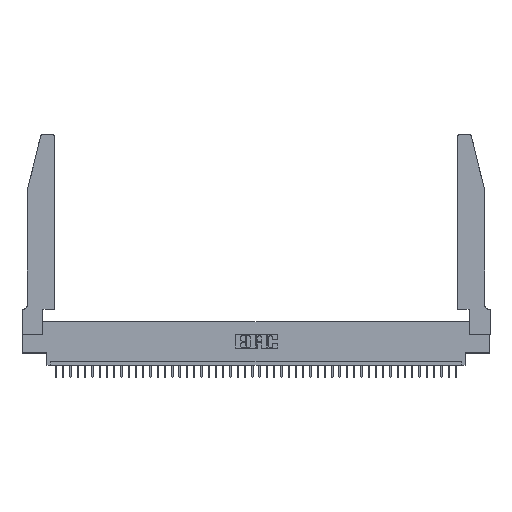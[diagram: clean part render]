
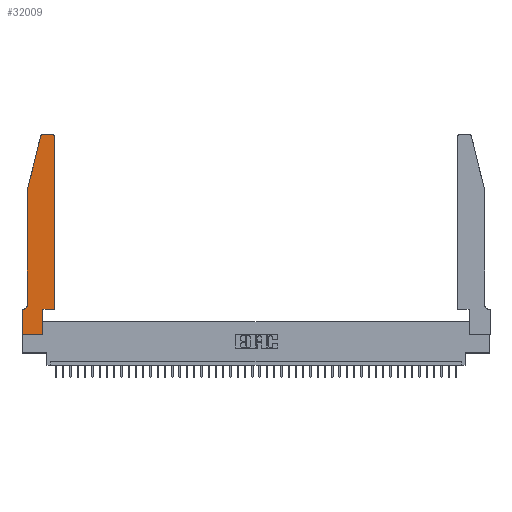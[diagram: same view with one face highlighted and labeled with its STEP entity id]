
A CAD part, top view. The second image highlights one B-rep face of the part: STEP entity #32009.
In plain terms, the highlighted planar face has unit normal (0, 0, 1).
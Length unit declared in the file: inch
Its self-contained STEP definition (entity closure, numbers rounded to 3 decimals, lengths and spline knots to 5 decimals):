
#18 = CARTESIAN_POINT ( 'NONE',  ( 0.0755, 0.42, 0.37 ) ) ;
#1356 = CIRCLE ( 'NONE', #8818, 0.07 ) ;
#1361 = EDGE_CURVE ( 'NONE', #44938, #2321, #7602, .T. ) ;
#1461 = CARTESIAN_POINT ( 'NONE',  ( 0., 0.35, 0.37 ) ) ;
#2094 = CARTESIAN_POINT ( 'NONE',  ( 0.0755, 0.35, 0.37 ) ) ;
#2321 = VERTEX_POINT ( 'NONE', #21608 ) ;
#2689 = VERTEX_POINT ( 'NONE', #36999 ) ;
#2797 = ORIENTED_EDGE ( 'NONE', *, *, #9534, .T. ) ;
#4117 = AXIS2_PLACEMENT_3D ( 'NONE', #1461, #36749, #15804 ) ;
#5917 = CARTESIAN_POINT ( 'NONE',  ( 0.4505, 2.72, 0.37 ) ) ;
#7086 = EDGE_CURVE ( 'NONE', #2689, #9109, #42545, .T. ) ;
#7531 = DIRECTION ( 'NONE',  ( 1., 0., 0. ) ) ;
#7602 = LINE ( 'NONE', #31807, #38711 ) ;
#7651 = EDGE_CURVE ( 'NONE', #26557, #43813, #8145, .T. ) ;
#8145 = LINE ( 'NONE', #15179, #40892 ) ;
#8818 = AXIS2_PLACEMENT_3D ( 'NONE', #43411, #18989, #39770 ) ;
#8921 = ORIENTED_EDGE ( 'NONE', *, *, #43146, .T. ) ;
#9109 = VERTEX_POINT ( 'NONE', #40360 ) ;
#9534 = EDGE_CURVE ( 'NONE', #9109, #19603, #30904, .T. ) ;
#10351 = CARTESIAN_POINT ( 'NONE',  ( 0.284, 2.75, 0.37 ) ) ;
#10446 = CARTESIAN_POINT ( 'NONE',  ( 0.4205, 2.75, 0.37 ) ) ;
#10692 = DIRECTION ( 'NONE',  ( 1., 0., 0. ) ) ;
#11407 = VECTOR ( 'NONE', #44811, 39.37008 ) ;
#11962 = ORIENTED_EDGE ( 'NONE', *, *, #36521, .T. ) ;
#12102 = EDGE_LOOP ( 'NONE', ( #14513, #35256, #32647, #8921, #28893, #36883, #13601, #25697, #11962, #14134, #2797, #15555 ) ) ;
#12489 = EDGE_CURVE ( 'NONE', #29312, #44938, #43324, .T. ) ;
#13601 = ORIENTED_EDGE ( 'NONE', *, *, #19888, .T. ) ;
#14099 = DIRECTION ( 'NONE',  ( 0., -1., 0. ) ) ;
#14134 = ORIENTED_EDGE ( 'NONE', *, *, #7086, .T. ) ;
#14513 = ORIENTED_EDGE ( 'NONE', *, *, #42113, .T. ) ;
#15005 = CARTESIAN_POINT ( 'NONE',  ( 0., 0., 0.37 ) ) ;
#15179 = CARTESIAN_POINT ( 'NONE',  ( 0., 0., 0.37 ) ) ;
#15311 = VERTEX_POINT ( 'NONE', #18 ) ;
#15555 = ORIENTED_EDGE ( 'NONE', *, *, #31331, .T. ) ;
#15804 = DIRECTION ( 'NONE',  ( 1., 0., 0. ) ) ;
#15891 = VERTEX_POINT ( 'NONE', #38110 ) ;
#15934 = DIRECTION ( 'NONE',  ( 0., 0., 1. ) ) ;
#16009 = CARTESIAN_POINT ( 'NONE',  ( 0.4505, 0.35, 0.37 ) ) ;
#16057 = LINE ( 'NONE', #15005, #42832 ) ;
#17105 = VECTOR ( 'NONE', #23163, 39.37008 ) ;
#17868 = DIRECTION ( 'NONE',  ( 0., 0., 1. ) ) ;
#18566 = DIRECTION ( 'NONE',  ( 1., 0., 0. ) ) ;
#18989 = DIRECTION ( 'NONE',  ( 0., 0., -1. ) ) ;
#19302 = VECTOR ( 'NONE', #24880, 39.37008 ) ;
#19389 = CARTESIAN_POINT ( 'NONE',  ( 0.0055, 0.35, 0.37 ) ) ;
#19603 = VERTEX_POINT ( 'NONE', #5917 ) ;
#19888 = EDGE_CURVE ( 'NONE', #15891, #26557, #16057, .T. ) ;
#20320 = EDGE_CURVE ( 'NONE', #27628, #15891, #25340, .T. ) ;
#21608 = CARTESIAN_POINT ( 'NONE',  ( 0.0755, 2., 0.37 ) ) ;
#22881 = LINE ( 'NONE', #26991, #11407 ) ;
#23163 = DIRECTION ( 'NONE',  ( -1., 0., 0. ) ) ;
#23839 = CARTESIAN_POINT ( 'NONE',  ( 0.2605, 2.75, 0.37 ) ) ;
#24000 = VERTEX_POINT ( 'NONE', #10446 ) ;
#24753 = CARTESIAN_POINT ( 'NONE',  ( 0.4505, 0.35, 0.37 ) ) ;
#24880 = DIRECTION ( 'NONE',  ( 0., 1., 0. ) ) ;
#25015 = CARTESIAN_POINT ( 'NONE',  ( 0.2865, 0.35, 0.37 ) ) ;
#25340 = LINE ( 'NONE', #2094, #17105 ) ;
#25630 = VECTOR ( 'NONE', #10692, 39.37008 ) ;
#25697 = ORIENTED_EDGE ( 'NONE', *, *, #7651, .T. ) ;
#25991 = VECTOR ( 'NONE', #40623, 39.37008 ) ;
#26242 = PLANE ( 'NONE',  #4117 ) ;
#26528 = DIRECTION ( 'NONE',  ( 1., 0., 0. ) ) ;
#26557 = VERTEX_POINT ( 'NONE', #40274 ) ;
#26742 = CARTESIAN_POINT ( 'NONE',  ( 0.2865, 0., 0.37 ) ) ;
#26991 = CARTESIAN_POINT ( 'NONE',  ( 0.0755, 2., 0.37 ) ) ;
#27628 = VERTEX_POINT ( 'NONE', #19389 ) ;
#28893 = ORIENTED_EDGE ( 'NONE', *, *, #44925, .T. ) ;
#29198 = AXIS2_PLACEMENT_3D ( 'NONE', #39396, #17868, #7531 ) ;
#29312 = VERTEX_POINT ( 'NONE', #10351 ) ;
#29405 = CARTESIAN_POINT ( 'NONE',  ( 0.25487, 2.72718, 0.37 ) ) ;
#30904 = LINE ( 'NONE', #16009, #25991 ) ;
#31331 = EDGE_CURVE ( 'NONE', #19603, #24000, #36213, .T. ) ;
#31357 = DIRECTION ( 'NONE',  ( -1., 0., 0. ) ) ;
#31807 = CARTESIAN_POINT ( 'NONE',  ( 0.0755, 2., 0.37 ) ) ;
#32009 = ADVANCED_FACE ( 'NONE', ( #37848 ), #26242, .T. ) ;
#32647 = ORIENTED_EDGE ( 'NONE', *, *, #1361, .T. ) ;
#33020 = VECTOR ( 'NONE', #31357, 39.37008 ) ;
#33562 = LINE ( 'NONE', #23839, #33020 ) ;
#35256 = ORIENTED_EDGE ( 'NONE', *, *, #12489, .T. ) ;
#36213 = CIRCLE ( 'NONE', #36898, 0.03 ) ;
#36521 = EDGE_CURVE ( 'NONE', #43813, #2689, #42244, .T. ) ;
#36749 = DIRECTION ( 'NONE',  ( 0., 0., 1. ) ) ;
#36883 = ORIENTED_EDGE ( 'NONE', *, *, #20320, .T. ) ;
#36898 = AXIS2_PLACEMENT_3D ( 'NONE', #43903, #15934, #26528 ) ;
#36999 = CARTESIAN_POINT ( 'NONE',  ( 0.2865, 0.35, 0.37 ) ) ;
#37848 = FACE_OUTER_BOUND ( 'NONE', #12102, .T. ) ;
#38110 = CARTESIAN_POINT ( 'NONE',  ( 0., 0.35, 0.37 ) ) ;
#38711 = VECTOR ( 'NONE', #43343, 39.37008 ) ;
#39396 = CARTESIAN_POINT ( 'NONE',  ( 0.284, 2.72, 0.37 ) ) ;
#39770 = DIRECTION ( 'NONE',  ( -1., 0., 0. ) ) ;
#40274 = CARTESIAN_POINT ( 'NONE',  ( 0., 0., 0.37 ) ) ;
#40360 = CARTESIAN_POINT ( 'NONE',  ( 0.4505, 0.35, 0.37 ) ) ;
#40623 = DIRECTION ( 'NONE',  ( 0., 1., 0. ) ) ;
#40892 = VECTOR ( 'NONE', #18566, 39.37008 ) ;
#42113 = EDGE_CURVE ( 'NONE', #24000, #29312, #33562, .T. ) ;
#42244 = LINE ( 'NONE', #25015, #19302 ) ;
#42545 = LINE ( 'NONE', #24753, #25630 ) ;
#42832 = VECTOR ( 'NONE', #14099, 39.37008 ) ;
#43146 = EDGE_CURVE ( 'NONE', #2321, #15311, #22881, .T. ) ;
#43324 = CIRCLE ( 'NONE', #29198, 0.03 ) ;
#43343 = DIRECTION ( 'NONE',  ( -0.239, -0.971, 0. ) ) ;
#43411 = CARTESIAN_POINT ( 'NONE',  ( 0.0055, 0.42, 0.37 ) ) ;
#43813 = VERTEX_POINT ( 'NONE', #26742 ) ;
#43903 = CARTESIAN_POINT ( 'NONE',  ( 0.4205, 2.72, 0.37 ) ) ;
#44811 = DIRECTION ( 'NONE',  ( 0., -1., 0. ) ) ;
#44925 = EDGE_CURVE ( 'NONE', #15311, #27628, #1356, .T. ) ;
#44938 = VERTEX_POINT ( 'NONE', #29405 ) ;
